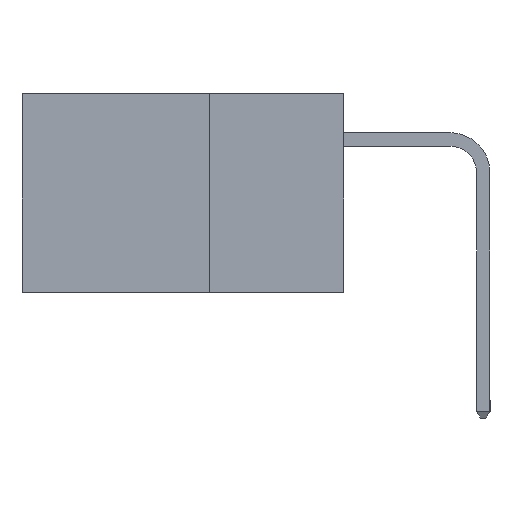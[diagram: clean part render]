
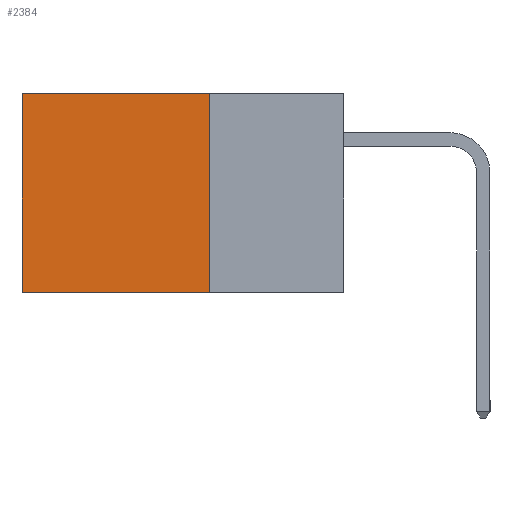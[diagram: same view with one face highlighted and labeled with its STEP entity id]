
A CAD part, left-side view. The second image highlights one B-rep face of the part: STEP entity #2384.
In plain terms, the highlighted planar face has unit normal (-1, 0, 0).
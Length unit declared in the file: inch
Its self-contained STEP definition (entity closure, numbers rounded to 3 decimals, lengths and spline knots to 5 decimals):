
#49 = EDGE_CURVE ( 'NONE', #1088, #4225, #15046, .T. ) ;
#345 = DIRECTION ( 'NONE',  ( 1., 0., 0. ) ) ;
#355 = DIRECTION ( 'NONE',  ( 0., 0., -1. ) ) ;
#397 = CARTESIAN_POINT ( 'NONE',  ( 0.2615, 0.25, -0.37 ) ) ;
#865 = EDGE_LOOP ( 'NONE', ( #6964, #7119, #7473, #8107 ) ) ;
#899 = PLANE ( 'NONE',  #12637 ) ;
#1069 = LINE ( 'NONE', #11671, #13189 ) ;
#1088 = VERTEX_POINT ( 'NONE', #2701 ) ;
#1264 = VECTOR ( 'NONE', #5066, 39.37008 ) ;
#2147 = CARTESIAN_POINT ( 'NONE',  ( 0.2615, 0.25, 0. ) ) ;
#2384 = ADVANCED_FACE ( 'NONE', ( #2466 ), #899, .F. ) ;
#2466 = FACE_OUTER_BOUND ( 'NONE', #865, .T. ) ;
#2574 = VERTEX_POINT ( 'NONE', #2147 ) ;
#2701 = CARTESIAN_POINT ( 'NONE',  ( 0.2615, 0.6, 0. ) ) ;
#3638 = CARTESIAN_POINT ( 'NONE',  ( 0.2615, 0.25, 0. ) ) ;
#4225 = VERTEX_POINT ( 'NONE', #14118 ) ;
#4719 = DIRECTION ( 'NONE',  ( 0., 1., 0. ) ) ;
#4858 = DIRECTION ( 'NONE',  ( 0., 1., 0. ) ) ;
#5066 = DIRECTION ( 'NONE',  ( 0., 0., -1. ) ) ;
#5948 = LINE ( 'NONE', #3638, #11729 ) ;
#6297 = VECTOR ( 'NONE', #355, 39.37008 ) ;
#6964 = ORIENTED_EDGE ( 'NONE', *, *, #49, .T. ) ;
#7119 = ORIENTED_EDGE ( 'NONE', *, *, #11853, .F. ) ;
#7211 = DIRECTION ( 'NONE',  ( 0., 0., -1. ) ) ;
#7248 = LINE ( 'NONE', #8537, #1264 ) ;
#7473 = ORIENTED_EDGE ( 'NONE', *, *, #11338, .F. ) ;
#8107 = ORIENTED_EDGE ( 'NONE', *, *, #12845, .T. ) ;
#8537 = CARTESIAN_POINT ( 'NONE',  ( 0.2615, 0.25, -0.37 ) ) ;
#8694 = CARTESIAN_POINT ( 'NONE',  ( 0.2615, 0.6, -0.37 ) ) ;
#9565 = CARTESIAN_POINT ( 'NONE',  ( 0.2615, 0.25, -0.37 ) ) ;
#11338 = EDGE_CURVE ( 'NONE', #2574, #12862, #7248, .T. ) ;
#11671 = CARTESIAN_POINT ( 'NONE',  ( 0.2615, 0.25, -0.37 ) ) ;
#11729 = VECTOR ( 'NONE', #4858, 39.37008 ) ;
#11853 = EDGE_CURVE ( 'NONE', #12862, #4225, #1069, .T. ) ;
#12637 = AXIS2_PLACEMENT_3D ( 'NONE', #397, #345, #7211 ) ;
#12845 = EDGE_CURVE ( 'NONE', #2574, #1088, #5948, .T. ) ;
#12862 = VERTEX_POINT ( 'NONE', #9565 ) ;
#13189 = VECTOR ( 'NONE', #4719, 39.37008 ) ;
#14118 = CARTESIAN_POINT ( 'NONE',  ( 0.2615, 0.6, -0.37 ) ) ;
#15046 = LINE ( 'NONE', #8694, #6297 ) ;
